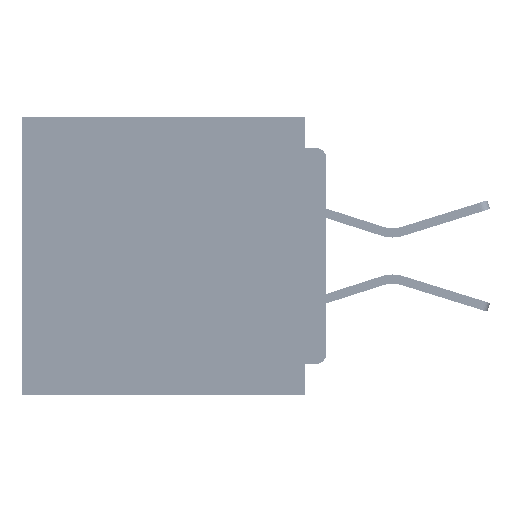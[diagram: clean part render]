
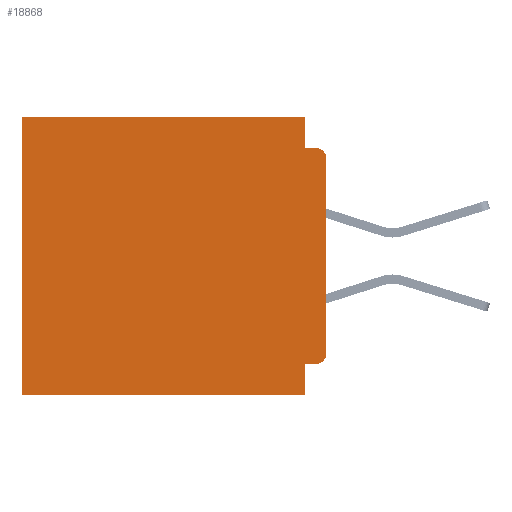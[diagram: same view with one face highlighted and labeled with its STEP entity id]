
A CAD part, left-side view. The second image highlights one B-rep face of the part: STEP entity #18868.
In plain terms, the highlighted planar face has unit normal (-1, 0, 0).
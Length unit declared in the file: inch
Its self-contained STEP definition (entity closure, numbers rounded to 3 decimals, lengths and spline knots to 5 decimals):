
#652 = CARTESIAN_POINT ( 'NONE',  ( 0.3, 0., -0.34 ) ) ;
#733 = CARTESIAN_POINT ( 'NONE',  ( 0.3, 0.031, 0. ) ) ;
#1223 = LINE ( 'NONE', #19062, #26391 ) ;
#1556 = ORIENTED_EDGE ( 'NONE', *, *, #48444, .F. ) ;
#3117 = CARTESIAN_POINT ( 'NONE',  ( 0.3, 0.015, -0.045 ) ) ;
#3376 = VECTOR ( 'NONE', #14762, 39.37008 ) ;
#3612 = VECTOR ( 'NONE', #51401, 39.37008 ) ;
#4674 = CARTESIAN_POINT ( 'NONE',  ( 0.3, 0., -0.355 ) ) ;
#8346 = EDGE_CURVE ( 'NONE', #9046, #46885, #46990, .T. ) ;
#9046 = VERTEX_POINT ( 'NONE', #733 ) ;
#9398 = DIRECTION ( 'NONE',  ( 0., 0., -1. ) ) ;
#10400 = VERTEX_POINT ( 'NONE', #41107 ) ;
#11713 = CARTESIAN_POINT ( 'NONE',  ( 0.3, 0.437, -0.4 ) ) ;
#11791 = VECTOR ( 'NONE', #54162, 39.37008 ) ;
#14762 = DIRECTION ( 'NONE',  ( 0., 1., 0. ) ) ;
#16958 = FACE_OUTER_BOUND ( 'NONE', #22728, .T. ) ;
#17243 = VECTOR ( 'NONE', #43217, 39.37008 ) ;
#17335 = ORIENTED_EDGE ( 'NONE', *, *, #43207, .F. ) ;
#17946 = EDGE_CURVE ( 'NONE', #10400, #28427, #20247, .T. ) ;
#18684 = CARTESIAN_POINT ( 'NONE',  ( 0.3, 0., -0.06 ) ) ;
#18868 = ADVANCED_FACE ( 'NONE', ( #16958 ), #42647, .F. ) ;
#19062 = CARTESIAN_POINT ( 'NONE',  ( 0.3, 0.437, -0.4 ) ) ;
#19758 = DIRECTION ( 'NONE',  ( 0., -1., 0. ) ) ;
#20247 = LINE ( 'NONE', #59641, #58435 ) ;
#20792 = CARTESIAN_POINT ( 'NONE',  ( 0.3, 0.015, -0.06 ) ) ;
#21550 = CARTESIAN_POINT ( 'NONE',  ( 0.3, 0.031, -0.4 ) ) ;
#22728 = EDGE_LOOP ( 'NONE', ( #51484, #55467, #50070, #1556, #39217, #22864, #37709, #17335, #25258, #29997 ) ) ;
#22864 = ORIENTED_EDGE ( 'NONE', *, *, #36506, .T. ) ;
#23037 = VERTEX_POINT ( 'NONE', #44198 ) ;
#24547 = VERTEX_POINT ( 'NONE', #652 ) ;
#24756 = CARTESIAN_POINT ( 'NONE',  ( 0.3, 0., -0.4 ) ) ;
#25197 = LINE ( 'NONE', #34219, #11791 ) ;
#25210 = CARTESIAN_POINT ( 'NONE',  ( 0.3, 0., 0. ) ) ;
#25258 = ORIENTED_EDGE ( 'NONE', *, *, #45683, .F. ) ;
#25877 = DIRECTION ( 'NONE',  ( 0., 0., -1. ) ) ;
#26239 = DIRECTION ( 'NONE',  ( -1., 0., 0. ) ) ;
#26316 = CARTESIAN_POINT ( 'NONE',  ( 0.3, 0.437, 0. ) ) ;
#26391 = VECTOR ( 'NONE', #9398, 39.37008 ) ;
#27829 = DIRECTION ( 'NONE',  ( 0., 0., -1. ) ) ;
#28408 = CARTESIAN_POINT ( 'NONE',  ( 0.3, 0., -0.4 ) ) ;
#28427 = VERTEX_POINT ( 'NONE', #3117 ) ;
#29997 = ORIENTED_EDGE ( 'NONE', *, *, #53608, .T. ) ;
#32222 = LINE ( 'NONE', #28408, #17243 ) ;
#33768 = VECTOR ( 'NONE', #54998, 39.37008 ) ;
#34219 = CARTESIAN_POINT ( 'NONE',  ( 0.3, 0.031, 0. ) ) ;
#34844 = EDGE_CURVE ( 'NONE', #63240, #28427, #39876, .T. ) ;
#35683 = LINE ( 'NONE', #24756, #50439 ) ;
#36506 = EDGE_CURVE ( 'NONE', #46885, #56236, #1223, .T. ) ;
#37709 = ORIENTED_EDGE ( 'NONE', *, *, #41071, .F. ) ;
#37883 = EDGE_CURVE ( 'NONE', #63240, #24547, #35683, .T. ) ;
#38533 = VERTEX_POINT ( 'NONE', #49932 ) ;
#39217 = ORIENTED_EDGE ( 'NONE', *, *, #8346, .T. ) ;
#39876 = CIRCLE ( 'NONE', #43290, 0.015 ) ;
#41071 = EDGE_CURVE ( 'NONE', #38533, #56236, #32222, .T. ) ;
#41107 = CARTESIAN_POINT ( 'NONE',  ( 0.3, 0.031, -0.045 ) ) ;
#42462 = LINE ( 'NONE', #4674, #3376 ) ;
#42647 = PLANE ( 'NONE',  #55339 ) ;
#43207 = EDGE_CURVE ( 'NONE', #62729, #38533, #56735, .T. ) ;
#43217 = DIRECTION ( 'NONE',  ( 0., 1., 0. ) ) ;
#43290 = AXIS2_PLACEMENT_3D ( 'NONE', #20792, #55654, #25877 ) ;
#44198 = CARTESIAN_POINT ( 'NONE',  ( 0.3, 0.015, -0.355 ) ) ;
#44612 = DIRECTION ( 'NONE',  ( 0., 0., -1. ) ) ;
#45683 = EDGE_CURVE ( 'NONE', #23037, #62729, #42462, .T. ) ;
#46885 = VERTEX_POINT ( 'NONE', #26316 ) ;
#46990 = LINE ( 'NONE', #25210, #33768 ) ;
#47288 = CIRCLE ( 'NONE', #58728, 0.015 ) ;
#48444 = EDGE_CURVE ( 'NONE', #9046, #10400, #25197, .T. ) ;
#49932 = CARTESIAN_POINT ( 'NONE',  ( 0.3, 0.031, -0.4 ) ) ;
#49973 = CARTESIAN_POINT ( 'NONE',  ( 0.3, 0.031, -0.355 ) ) ;
#50070 = ORIENTED_EDGE ( 'NONE', *, *, #17946, .F. ) ;
#50439 = VECTOR ( 'NONE', #44612, 39.37008 ) ;
#51401 = DIRECTION ( 'NONE',  ( 0., 0., -1. ) ) ;
#51484 = ORIENTED_EDGE ( 'NONE', *, *, #37883, .F. ) ;
#52582 = CARTESIAN_POINT ( 'NONE',  ( 0.3, 0., -0.4 ) ) ;
#53608 = EDGE_CURVE ( 'NONE', #23037, #24547, #47288, .T. ) ;
#54162 = DIRECTION ( 'NONE',  ( 0., 0., -1. ) ) ;
#54998 = DIRECTION ( 'NONE',  ( 0., 1., 0. ) ) ;
#55339 = AXIS2_PLACEMENT_3D ( 'NONE', #52582, #57561, #27829 ) ;
#55467 = ORIENTED_EDGE ( 'NONE', *, *, #34844, .T. ) ;
#55654 = DIRECTION ( 'NONE',  ( -1., 0., 0. ) ) ;
#55997 = CARTESIAN_POINT ( 'NONE',  ( 0.3, 0.015, -0.34 ) ) ;
#56236 = VERTEX_POINT ( 'NONE', #11713 ) ;
#56735 = LINE ( 'NONE', #21550, #3612 ) ;
#57561 = DIRECTION ( 'NONE',  ( 1., 0., 0. ) ) ;
#58435 = VECTOR ( 'NONE', #19758, 39.37008 ) ;
#58728 = AXIS2_PLACEMENT_3D ( 'NONE', #55997, #26239, #61015 ) ;
#59641 = CARTESIAN_POINT ( 'NONE',  ( 0.3, 0., -0.045 ) ) ;
#61015 = DIRECTION ( 'NONE',  ( 0., 0., -1. ) ) ;
#62729 = VERTEX_POINT ( 'NONE', #49973 ) ;
#63240 = VERTEX_POINT ( 'NONE', #18684 ) ;
